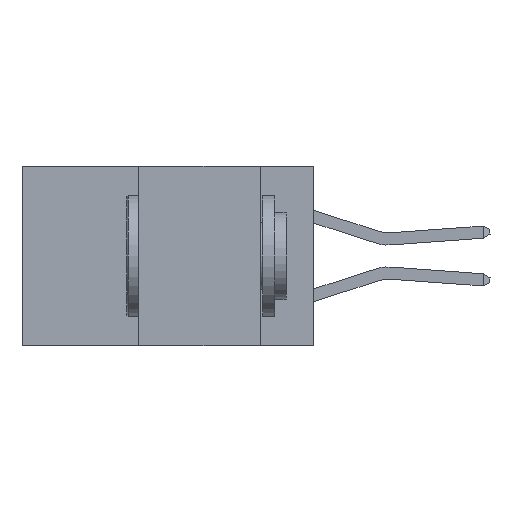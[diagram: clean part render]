
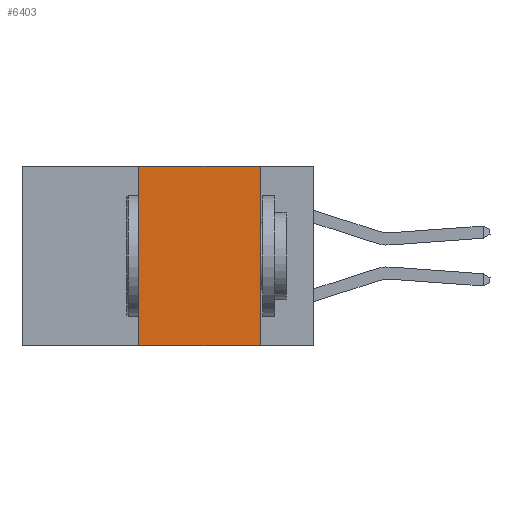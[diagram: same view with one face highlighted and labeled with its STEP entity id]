
A CAD part, left-side view. The second image highlights one B-rep face of the part: STEP entity #6403.
In plain terms, the highlighted planar face has unit normal (-1, 0, 0).
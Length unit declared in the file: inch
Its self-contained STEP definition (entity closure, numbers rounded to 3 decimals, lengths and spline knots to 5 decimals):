
#1638 = CARTESIAN_POINT ( 'NONE',  ( 0., 0.11, 0. ) ) ;
#3317 = DIRECTION ( 'NONE',  ( 0., 0., 1. ) ) ;
#4157 = CARTESIAN_POINT ( 'NONE',  ( 0., 0.6, 0. ) ) ;
#4521 = DIRECTION ( 'NONE',  ( 0., 0., -1. ) ) ;
#5059 = EDGE_CURVE ( 'NONE', #20746, #29671, #7739, .T. ) ;
#6403 = ADVANCED_FACE ( 'NONE', ( #35973 ), #24352, .F. ) ;
#6891 = CARTESIAN_POINT ( 'NONE',  ( 0., 0.11, 0. ) ) ;
#7408 = VERTEX_POINT ( 'NONE', #1638 ) ;
#7739 = LINE ( 'NONE', #35234, #20740 ) ;
#8017 = ORIENTED_EDGE ( 'NONE', *, *, #35955, .F. ) ;
#8840 = AXIS2_PLACEMENT_3D ( 'NONE', #33901, #31166, #31282 ) ;
#9667 = LINE ( 'NONE', #4157, #14145 ) ;
#11036 = ORIENTED_EDGE ( 'NONE', *, *, #25253, .F. ) ;
#14145 = VECTOR ( 'NONE', #18492, 39.37008 ) ;
#15775 = LINE ( 'NONE', #6891, #30967 ) ;
#16725 = VERTEX_POINT ( 'NONE', #27411 ) ;
#17747 = EDGE_LOOP ( 'NONE', ( #27537, #11036, #8017, #31135 ) ) ;
#18492 = DIRECTION ( 'NONE',  ( 0., -1., 0. ) ) ;
#20740 = VECTOR ( 'NONE', #23397, 39.37008 ) ;
#20746 = VERTEX_POINT ( 'NONE', #29609 ) ;
#20752 = CARTESIAN_POINT ( 'NONE',  ( 0., 0.11, -0.37 ) ) ;
#23397 = DIRECTION ( 'NONE',  ( 0., -1., 0. ) ) ;
#24352 = PLANE ( 'NONE',  #8840 ) ;
#25253 = EDGE_CURVE ( 'NONE', #16725, #7408, #9667, .T. ) ;
#26782 = EDGE_CURVE ( 'NONE', #7408, #29671, #15775, .T. ) ;
#27411 = CARTESIAN_POINT ( 'NONE',  ( 0., 0.36, 0. ) ) ;
#27537 = ORIENTED_EDGE ( 'NONE', *, *, #26782, .F. ) ;
#27828 = VECTOR ( 'NONE', #3317, 39.37008 ) ;
#29609 = CARTESIAN_POINT ( 'NONE',  ( 0., 0.36, -0.37 ) ) ;
#29671 = VERTEX_POINT ( 'NONE', #20752 ) ;
#30967 = VECTOR ( 'NONE', #4521, 39.37008 ) ;
#31135 = ORIENTED_EDGE ( 'NONE', *, *, #5059, .T. ) ;
#31166 = DIRECTION ( 'NONE',  ( 1., 0., 0. ) ) ;
#31282 = DIRECTION ( 'NONE',  ( 0., 0., -1. ) ) ;
#31850 = CARTESIAN_POINT ( 'NONE',  ( 0., 0.36, 0. ) ) ;
#33901 = CARTESIAN_POINT ( 'NONE',  ( 0., 0.6, 0. ) ) ;
#35234 = CARTESIAN_POINT ( 'NONE',  ( 0., 0.6, -0.37 ) ) ;
#35350 = LINE ( 'NONE', #31850, #27828 ) ;
#35955 = EDGE_CURVE ( 'NONE', #20746, #16725, #35350, .T. ) ;
#35973 = FACE_OUTER_BOUND ( 'NONE', #17747, .T. ) ;
